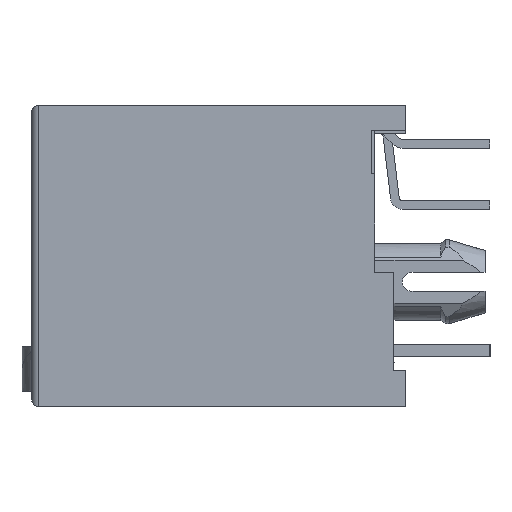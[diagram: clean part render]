
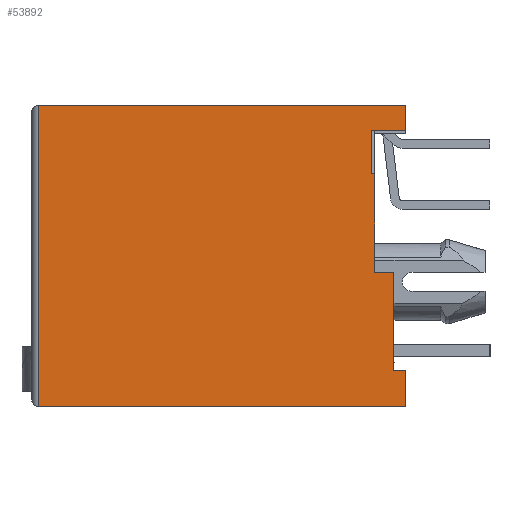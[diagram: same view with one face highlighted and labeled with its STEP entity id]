
A CAD part, left-side view. The second image highlights one B-rep face of the part: STEP entity #53892.
In plain terms, the highlighted planar face has unit normal (-1, 0, 0).
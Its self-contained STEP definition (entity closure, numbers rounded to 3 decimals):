
#89 = CARTESIAN_POINT ( 'NONE',  ( -31.5, 7.5, 6.3 ) ) ;
#499 = CARTESIAN_POINT ( 'NONE',  ( -31.5, -6.767, -0.65 ) ) ;
#1816 = DIRECTION ( 'NONE',  ( 0., 0., 1. ) ) ;
#2936 = CARTESIAN_POINT ( 'NONE',  ( -31.5, -6.35, 3.45 ) ) ;
#3133 = VERTEX_POINT ( 'NONE', #11465 ) ;
#3209 = B_SPLINE_CURVE_WITH_KNOTS ( 'NONE', 3,
 ( #59203, #10475, #32139, #53850 ),
 .UNSPECIFIED., .F., .F.,
 ( 4, 4 ),
 ( 0., 1. ),
 .UNSPECIFIED. ) ;
#4014 = VERTEX_POINT ( 'NONE', #18020 ) ;
#5438 = CARTESIAN_POINT ( 'NONE',  ( -31.5, -7.8, -6.25 ) ) ;
#5904 = VERTEX_POINT ( 'NONE', #5438 ) ;
#6218 = CARTESIAN_POINT ( 'NONE',  ( -31.5, -2.7, -6.25 ) ) ;
#6406 = VERTEX_POINT ( 'NONE', #21084 ) ;
#6780 = EDGE_CURVE ( 'NONE', #64469, #5904, #18770, .T. ) ;
#7841 = CARTESIAN_POINT ( 'NONE',  ( -31.5, 7.5, 6.3 ) ) ;
#8474 = EDGE_CURVE ( 'NONE', #21009, #33893, #3209, .T. ) ;
#8478 = CARTESIAN_POINT ( 'NONE',  ( -31.5, -7.633, -4.75 ) ) ;
#9126 = ORIENTED_EDGE ( 'NONE', *, *, #27507, .F. ) ;
#9518 = ORIENTED_EDGE ( 'NONE', *, *, #6780, .F. ) ;
#9534 = EDGE_CURVE ( 'NONE', #22850, #21009, #68341, .T. ) ;
#9737 = CARTESIAN_POINT ( 'NONE',  ( -31.5, -6.35, 3.45 ) ) ;
#10236 = CARTESIAN_POINT ( 'NONE',  ( -31.5, -7.8, 5.25 ) ) ;
#10246 = ORIENTED_EDGE ( 'NONE', *, *, #9534, .F. ) ;
#10475 = CARTESIAN_POINT ( 'NONE',  ( -31.5, -7.3, -2.017 ) ) ;
#11465 = CARTESIAN_POINT ( 'NONE',  ( -31.5, -6.5, 3.45 ) ) ;
#11485 = B_SPLINE_CURVE_WITH_KNOTS ( 'NONE', 3,
 ( #65600, #36805, #69537, #58874 ),
 .UNSPECIFIED., .F., .F.,
 ( 4, 4 ),
 ( 0., 1. ),
 .UNSPECIFIED. ) ;
#11686 = CARTESIAN_POINT ( 'NONE',  ( -31.5, -7.8, -5.25 ) ) ;
#12020 = VERTEX_POINT ( 'NONE', #42769 ) ;
#12343 = ORIENTED_EDGE ( 'NONE', *, *, #68616, .T. ) ;
#12738 = CARTESIAN_POINT ( 'NONE',  ( -31.5, -7.8, -4.75 ) ) ;
#14410 = VERTEX_POINT ( 'NONE', #36069 ) ;
#14659 = CARTESIAN_POINT ( 'NONE',  ( -31.5, -6.45, 3.45 ) ) ;
#17914 = CARTESIAN_POINT ( 'NONE',  ( -31.5, -7.3, -0.65 ) ) ;
#18020 = CARTESIAN_POINT ( 'NONE',  ( -31.5, -6.35, 5.25 ) ) ;
#18770 = B_SPLINE_CURVE_WITH_KNOTS ( 'NONE', 3,
 ( #12738, #11686, #33335, #60777 ),
 .UNSPECIFIED., .F., .F.,
 ( 4, 4 ),
 ( 0., 1. ),
 .UNSPECIFIED. ) ;
#20035 = CARTESIAN_POINT ( 'NONE',  ( -31.5, -6.35, 4.05 ) ) ;
#20273 = EDGE_CURVE ( 'NONE', #3133, #22850, #40895, .T. ) ;
#21009 = VERTEX_POINT ( 'NONE', #22918 ) ;
#21084 = CARTESIAN_POINT ( 'NONE',  ( -31.5, -6.35, 3.45 ) ) ;
#21308 = VERTEX_POINT ( 'NONE', #89 ) ;
#22573 = B_SPLINE_CURVE_WITH_KNOTS ( 'NONE', 3,
 ( #50923, #51983, #46290, #68020 ),
 .UNSPECIFIED., .F., .F.,
 ( 4, 4 ),
 ( 0., 1. ),
 .UNSPECIFIED. ) ;
#22850 = VERTEX_POINT ( 'NONE', #40519 ) ;
#22918 = CARTESIAN_POINT ( 'NONE',  ( -31.5, -7.3, -0.65 ) ) ;
#23094 = B_SPLINE_CURVE_WITH_KNOTS ( 'NONE', 3,
 ( #56218, #55859, #67241, #7841 ),
 .UNSPECIFIED., .F., .F.,
 ( 4, 4 ),
 ( 0., 1. ),
 .UNSPECIFIED. ) ;
#24331 = ORIENTED_EDGE ( 'NONE', *, *, #34483, .F. ) ;
#25458 = VERTEX_POINT ( 'NONE', #56226 ) ;
#25983 = B_SPLINE_CURVE_WITH_KNOTS ( 'NONE', 3,
 ( #69133, #48470, #20035, #9737 ),
 .UNSPECIFIED., .F., .F.,
 ( 4, 4 ),
 ( 0., 1. ),
 .UNSPECIFIED. ) ;
#27507 = EDGE_CURVE ( 'NONE', #5904, #14410, #47247, .T. ) ;
#28840 = CARTESIAN_POINT ( 'NONE',  ( -31.5, 7.806, -6.501 ) ) ;
#29852 = CARTESIAN_POINT ( 'NONE',  ( -31.5, -6.5, 0.717 ) ) ;
#30825 = ORIENTED_EDGE ( 'NONE', *, *, #8474, .F. ) ;
#30834 = CARTESIAN_POINT ( 'NONE',  ( -31.5, -7.467, -4.75 ) ) ;
#31150 = EDGE_CURVE ( 'NONE', #25458, #21308, #23094, .T. ) ;
#32139 = CARTESIAN_POINT ( 'NONE',  ( -31.5, -7.3, -3.383 ) ) ;
#33335 = CARTESIAN_POINT ( 'NONE',  ( -31.5, -7.8, -5.75 ) ) ;
#33893 = VERTEX_POINT ( 'NONE', #63946 ) ;
#34080 = EDGE_CURVE ( 'NONE', #12020, #4014, #44593, .T. ) ;
#34483 = EDGE_CURVE ( 'NONE', #25458, #12020, #11485, .T. ) ;
#35868 = CARTESIAN_POINT ( 'NONE',  ( -31.5, -6.5, -0.65 ) ) ;
#36069 = CARTESIAN_POINT ( 'NONE',  ( -31.5, 7.5, -6.25 ) ) ;
#36279 = ORIENTED_EDGE ( 'NONE', *, *, #50468, .F. ) ;
#36805 = CARTESIAN_POINT ( 'NONE',  ( -31.5, -7.8, 5.95 ) ) ;
#36993 = ORIENTED_EDGE ( 'NONE', *, *, #31150, .T. ) ;
#38793 = PLANE ( 'NONE',  #47845 ) ;
#38863 = B_SPLINE_CURVE_WITH_KNOTS ( 'NONE', 3,
 ( #2936, #46994, #14659, #69068 ),
 .UNSPECIFIED., .F., .F.,
 ( 4, 4 ),
 ( 0., 1. ),
 .UNSPECIFIED. ) ;
#40372 = ORIENTED_EDGE ( 'NONE', *, *, #20273, .F. ) ;
#40519 = CARTESIAN_POINT ( 'NONE',  ( -31.5, -6.5, -0.65 ) ) ;
#40523 = CARTESIAN_POINT ( 'NONE',  ( -31.5, -6.5, 2.083 ) ) ;
#40895 = B_SPLINE_CURVE_WITH_KNOTS ( 'NONE', 3,
 ( #46543, #40523, #29852, #35868 ),
 .UNSPECIFIED., .F., .F.,
 ( 4, 4 ),
 ( 0., 1. ),
 .UNSPECIFIED. ) ;
#41515 = CARTESIAN_POINT ( 'NONE',  ( -31.5, -7.8, -4.75 ) ) ;
#42769 = CARTESIAN_POINT ( 'NONE',  ( -31.5, -7.8, 5.25 ) ) ;
#43267 = CARTESIAN_POINT ( 'NONE',  ( -31.5, -6.35, 5.25 ) ) ;
#43888 = CARTESIAN_POINT ( 'NONE',  ( -31.5, 2.4, -6.25 ) ) ;
#44593 = B_SPLINE_CURVE_WITH_KNOTS ( 'NONE', 3,
 ( #10236, #70315, #53611, #43267 ),
 .UNSPECIFIED., .F., .F.,
 ( 4, 4 ),
 ( 0., 1. ),
 .UNSPECIFIED. ) ;
#45187 = FACE_OUTER_BOUND ( 'NONE', #68984, .T. ) ;
#45242 = CARTESIAN_POINT ( 'NONE',  ( -31.5, -7.8, -4.75 ) ) ;
#46290 = CARTESIAN_POINT ( 'NONE',  ( -31.5, 7.5, -2.067 ) ) ;
#46543 = CARTESIAN_POINT ( 'NONE',  ( -31.5, -6.5, 3.45 ) ) ;
#46994 = CARTESIAN_POINT ( 'NONE',  ( -31.5, -6.4, 3.45 ) ) ;
#47204 = ORIENTED_EDGE ( 'NONE', *, *, #68324, .F. ) ;
#47247 = B_SPLINE_CURVE_WITH_KNOTS ( 'NONE', 3,
 ( #60305, #6218, #43888, #64560 ),
 .UNSPECIFIED., .F., .F.,
 ( 4, 4 ),
 ( 0., 1. ),
 .UNSPECIFIED. ) ;
#47845 = AXIS2_PLACEMENT_3D ( 'NONE', #28840, #55879, #1816 ) ;
#48470 = CARTESIAN_POINT ( 'NONE',  ( -31.5, -6.35, 4.65 ) ) ;
#48641 = B_SPLINE_CURVE_WITH_KNOTS ( 'NONE', 3,
 ( #63589, #30834, #8478, #41515 ),
 .UNSPECIFIED., .F., .F.,
 ( 4, 4 ),
 ( 0., 1. ),
 .UNSPECIFIED. ) ;
#50468 = EDGE_CURVE ( 'NONE', #33893, #64469, #48641, .T. ) ;
#50923 = CARTESIAN_POINT ( 'NONE',  ( -31.5, 7.5, 6.3 ) ) ;
#51983 = CARTESIAN_POINT ( 'NONE',  ( -31.5, 7.5, 2.117 ) ) ;
#53611 = CARTESIAN_POINT ( 'NONE',  ( -31.5, -6.833, 5.25 ) ) ;
#53850 = CARTESIAN_POINT ( 'NONE',  ( -31.5, -7.3, -4.75 ) ) ;
#53892 = ADVANCED_FACE ( 'NONE', ( #45187 ), #38793, .F. ) ;
#54560 = CARTESIAN_POINT ( 'NONE',  ( -31.5, -6.5, -0.65 ) ) ;
#55859 = CARTESIAN_POINT ( 'NONE',  ( -31.5, -2.7, 6.3 ) ) ;
#55879 = DIRECTION ( 'NONE',  ( 1., 0., 0. ) ) ;
#56218 = CARTESIAN_POINT ( 'NONE',  ( -31.5, -7.8, 6.3 ) ) ;
#56226 = CARTESIAN_POINT ( 'NONE',  ( -31.5, -7.8, 6.3 ) ) ;
#57880 = ORIENTED_EDGE ( 'NONE', *, *, #62069, .F. ) ;
#58874 = CARTESIAN_POINT ( 'NONE',  ( -31.5, -7.8, 5.25 ) ) ;
#59203 = CARTESIAN_POINT ( 'NONE',  ( -31.5, -7.3, -0.65 ) ) ;
#60305 = CARTESIAN_POINT ( 'NONE',  ( -31.5, -7.8, -6.25 ) ) ;
#60777 = CARTESIAN_POINT ( 'NONE',  ( -31.5, -7.8, -6.25 ) ) ;
#62069 = EDGE_CURVE ( 'NONE', #6406, #3133, #38863, .T. ) ;
#63589 = CARTESIAN_POINT ( 'NONE',  ( -31.5, -7.3, -4.75 ) ) ;
#63946 = CARTESIAN_POINT ( 'NONE',  ( -31.5, -7.3, -4.75 ) ) ;
#64135 = ORIENTED_EDGE ( 'NONE', *, *, #34080, .F. ) ;
#64469 = VERTEX_POINT ( 'NONE', #45242 ) ;
#64560 = CARTESIAN_POINT ( 'NONE',  ( -31.5, 7.5, -6.25 ) ) ;
#65232 = CARTESIAN_POINT ( 'NONE',  ( -31.5, -7.033, -0.65 ) ) ;
#65600 = CARTESIAN_POINT ( 'NONE',  ( -31.5, -7.8, 6.3 ) ) ;
#67241 = CARTESIAN_POINT ( 'NONE',  ( -31.5, 2.4, 6.3 ) ) ;
#68020 = CARTESIAN_POINT ( 'NONE',  ( -31.5, 7.5, -6.25 ) ) ;
#68324 = EDGE_CURVE ( 'NONE', #4014, #6406, #25983, .T. ) ;
#68341 = B_SPLINE_CURVE_WITH_KNOTS ( 'NONE', 3,
 ( #54560, #499, #65232, #17914 ),
 .UNSPECIFIED., .F., .F.,
 ( 4, 4 ),
 ( 0., 1. ),
 .UNSPECIFIED. ) ;
#68616 = EDGE_CURVE ( 'NONE', #21308, #14410, #22573, .T. ) ;
#68984 = EDGE_LOOP ( 'NONE', ( #9518, #36279, #30825, #10246, #40372, #57880, #47204, #64135, #24331, #36993, #12343, #9126 ) ) ;
#69068 = CARTESIAN_POINT ( 'NONE',  ( -31.5, -6.5, 3.45 ) ) ;
#69133 = CARTESIAN_POINT ( 'NONE',  ( -31.5, -6.35, 5.25 ) ) ;
#69537 = CARTESIAN_POINT ( 'NONE',  ( -31.5, -7.8, 5.6 ) ) ;
#70315 = CARTESIAN_POINT ( 'NONE',  ( -31.5, -7.317, 5.25 ) ) ;
